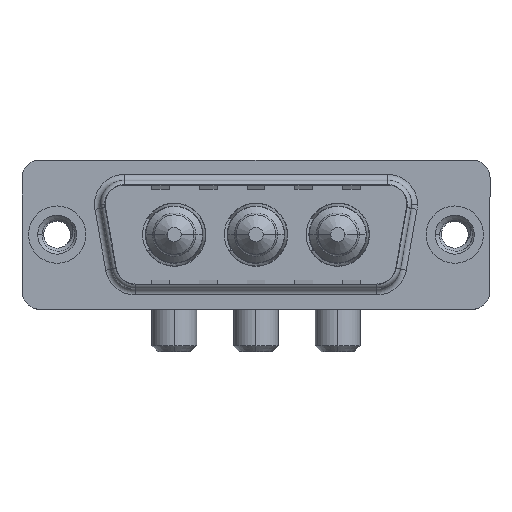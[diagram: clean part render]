
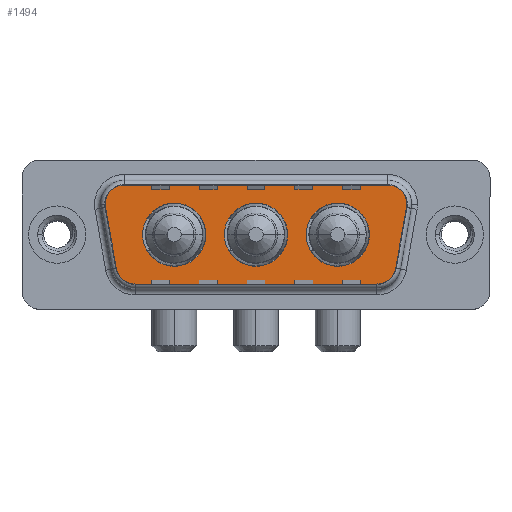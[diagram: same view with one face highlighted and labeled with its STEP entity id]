
A CAD part, top view. The second image highlights one B-rep face of the part: STEP entity #1494.
In plain terms, the highlighted planar face has unit normal (0, 0, 1).
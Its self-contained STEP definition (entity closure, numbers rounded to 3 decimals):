
#97 = ORIENTED_EDGE ( 'NONE', *, *, #5931, .T. ) ;
#112 = EDGE_LOOP ( 'NONE', ( #802, #237 ) ) ;
#126 = ORIENTED_EDGE ( 'NONE', *, *, #7953, .T. ) ;
#143 = CIRCLE ( 'NONE', #6179, 2.65 ) ;
#225 = FACE_BOUND ( 'NONE', #112, .T. ) ;
#237 = ORIENTED_EDGE ( 'NONE', *, *, #694, .F. ) ;
#276 = ORIENTED_EDGE ( 'NONE', *, *, #11775, .F. ) ;
#366 = EDGE_CURVE ( 'NONE', #3115, #2469, #8576, .T. ) ;
#438 = DIRECTION ( 'NONE',  ( 0., 0., 1. ) ) ;
#496 = CARTESIAN_POINT ( 'NONE',  ( 26.866, -2.9, 0. ) ) ;
#541 = CIRCLE ( 'NONE', #2817, 2. ) ;
#557 = DIRECTION ( 'NONE',  ( 1., 0., 0. ) ) ;
#694 = EDGE_CURVE ( 'NONE', #3726, #1870, #6298, .T. ) ;
#802 = ORIENTED_EDGE ( 'NONE', *, *, #11049, .F. ) ;
#808 = CARTESIAN_POINT ( 'NONE',  ( 23.5, 0., 0. ) ) ;
#925 = FACE_BOUND ( 'NONE', #8384, .T. ) ;
#1011 = CARTESIAN_POINT ( 'NONE',  ( 29.859, 2.553, 0. ) ) ;
#1080 = CIRCLE ( 'NONE', #6292, 2. ) ;
#1081 = CARTESIAN_POINT ( 'NONE',  ( 4.464, -3.247, 0. ) ) ;
#1180 = ORIENTED_EDGE ( 'NONE', *, *, #366, .T. ) ;
#1191 = CARTESIAN_POINT ( 'NONE',  ( 26.866, -2.9, 0. ) ) ;
#1372 = DIRECTION ( 'NONE',  ( 0., 0., 1. ) ) ;
#1472 = DIRECTION ( 'NONE',  ( 1., 0., 0. ) ) ;
#1494 = ADVANCED_FACE ( 'NONE', ( #10146, #925, #225, #2933 ), #9034, .T. ) ;
#1510 = ORIENTED_EDGE ( 'NONE', *, *, #2266, .T. ) ;
#1713 = AXIS2_PLACEMENT_3D ( 'NONE', #1191, #9162, #8184 ) ;
#1784 = AXIS2_PLACEMENT_3D ( 'NONE', #7742, #1927, #6703 ) ;
#1803 = AXIS2_PLACEMENT_3D ( 'NONE', #6799, #9805, #8179 ) ;
#1870 = VERTEX_POINT ( 'NONE', #9082 ) ;
#1927 = DIRECTION ( 'NONE',  ( 0., 0., 1. ) ) ;
#1985 = ORIENTED_EDGE ( 'NONE', *, *, #9459, .F. ) ;
#2036 = CARTESIAN_POINT ( 'NONE',  ( 27.889, 4.9, 0. ) ) ;
#2051 = VERTEX_POINT ( 'NONE', #4341 ) ;
#2266 = EDGE_CURVE ( 'NONE', #2051, #5206, #11802, .T. ) ;
#2469 = VERTEX_POINT ( 'NONE', #2036 ) ;
#2501 = DIRECTION ( 'NONE',  ( 0., 0., 1. ) ) ;
#2682 = DIRECTION ( 'NONE',  ( 0.174, -0.985, 0. ) ) ;
#2817 = AXIS2_PLACEMENT_3D ( 'NONE', #11311, #12238, #8225 ) ;
#2933 = FACE_OUTER_BOUND ( 'NONE', #5765, .T. ) ;
#2981 = CARTESIAN_POINT ( 'NONE',  ( 5.411, 4.9, 0. ) ) ;
#2986 = CARTESIAN_POINT ( 'NONE',  ( 5.411, 2.9, 0. ) ) ;
#3115 = VERTEX_POINT ( 'NONE', #12244 ) ;
#3294 = AXIS2_PLACEMENT_3D ( 'NONE', #808, #12917, #5832 ) ;
#3415 = VECTOR ( 'NONE', #2682, 1000. ) ;
#3726 = VERTEX_POINT ( 'NONE', #6502 ) ;
#4155 = DIRECTION ( 'NONE',  ( 0., 0., 1. ) ) ;
#4234 = EDGE_CURVE ( 'NONE', #7872, #2051, #11954, .T. ) ;
#4341 = CARTESIAN_POINT ( 'NONE',  ( 3.441, 2.553, 0. ) ) ;
#4369 = CARTESIAN_POINT ( 'NONE',  ( 20.85, 0., 0. ) ) ;
#4537 = DIRECTION ( 'NONE',  ( 1., 0., 0. ) ) ;
#4610 = ORIENTED_EDGE ( 'NONE', *, *, #10403, .T. ) ;
#4778 = VERTEX_POINT ( 'NONE', #6060 ) ;
#5125 = CIRCLE ( 'NONE', #6165, 2.65 ) ;
#5206 = VERTEX_POINT ( 'NONE', #1081 ) ;
#5215 = DIRECTION ( 'NONE',  ( -1., 0., 0. ) ) ;
#5291 = CARTESIAN_POINT ( 'NONE',  ( 27.889, 2.9, 0. ) ) ;
#5457 = EDGE_CURVE ( 'NONE', #4778, #12009, #1080, .T. ) ;
#5512 = CARTESIAN_POINT ( 'NONE',  ( 6.434, -4.9, 0. ) ) ;
#5677 = VECTOR ( 'NONE', #12750, 1000. ) ;
#5765 = EDGE_LOOP ( 'NONE', ( #12275, #97, #8215, #1180, #126, #8642, #1510, #4610, #12386 ) ) ;
#5774 = VECTOR ( 'NONE', #557, 1000. ) ;
#5832 = DIRECTION ( 'NONE',  ( 1., 0., 0. ) ) ;
#5931 = EDGE_CURVE ( 'NONE', #12009, #6503, #7456, .T. ) ;
#6060 = CARTESIAN_POINT ( 'NONE',  ( 26.866, -4.9, 0. ) ) ;
#6165 = AXIS2_PLACEMENT_3D ( 'NONE', #9311, #2501, #8082 ) ;
#6179 = AXIS2_PLACEMENT_3D ( 'NONE', #11361, #12417, #4537 ) ;
#6241 = DIRECTION ( 'NONE',  ( 1., 0., 0. ) ) ;
#6292 = AXIS2_PLACEMENT_3D ( 'NONE', #496, #11485, #12654 ) ;
#6298 = CIRCLE ( 'NONE', #6494, 2.65 ) ;
#6391 = CIRCLE ( 'NONE', #1784, 2. ) ;
#6456 = ORIENTED_EDGE ( 'NONE', *, *, #12552, .F. ) ;
#6476 = CARTESIAN_POINT ( 'NONE',  ( 29.859, 2.553, 0. ) ) ;
#6494 = AXIS2_PLACEMENT_3D ( 'NONE', #9323, #438, #1472 ) ;
#6502 = CARTESIAN_POINT ( 'NONE',  ( 7.15, 0., 0. ) ) ;
#6503 = VERTEX_POINT ( 'NONE', #1011 ) ;
#6703 = DIRECTION ( 'NONE',  ( -1., 0., 0. ) ) ;
#6799 = CARTESIAN_POINT ( 'NONE',  ( 23.5, 0., 0. ) ) ;
#6870 = EDGE_LOOP ( 'NONE', ( #1985, #7999 ) ) ;
#7189 = VERTEX_POINT ( 'NONE', #8636 ) ;
#7347 = LINE ( 'NONE', #5512, #5774 ) ;
#7456 = LINE ( 'NONE', #6476, #5677 ) ;
#7674 = CIRCLE ( 'NONE', #3294, 2.65 ) ;
#7742 = CARTESIAN_POINT ( 'NONE',  ( 27.889, 2.9, 0. ) ) ;
#7860 = VERTEX_POINT ( 'NONE', #11845 ) ;
#7872 = VERTEX_POINT ( 'NONE', #2981 ) ;
#7953 = EDGE_CURVE ( 'NONE', #2469, #7872, #11120, .T. ) ;
#7999 = ORIENTED_EDGE ( 'NONE', *, *, #8372, .F. ) ;
#8019 = VERTEX_POINT ( 'NONE', #4369 ) ;
#8031 = DIRECTION ( 'NONE',  ( 1., 0., 0. ) ) ;
#8082 = DIRECTION ( 'NONE',  ( 1., 0., 0. ) ) ;
#8141 = CARTESIAN_POINT ( 'NONE',  ( 16.65, 0., 0. ) ) ;
#8162 = CARTESIAN_POINT ( 'NONE',  ( 5.411, 4.9, 0. ) ) ;
#8179 = DIRECTION ( 'NONE',  ( 1., 0., 0. ) ) ;
#8184 = DIRECTION ( 'NONE',  ( 1., 0., 0. ) ) ;
#8215 = ORIENTED_EDGE ( 'NONE', *, *, #10777, .T. ) ;
#8225 = DIRECTION ( 'NONE',  ( -1., 0., 0. ) ) ;
#8372 = EDGE_CURVE ( 'NONE', #7189, #7860, #5125, .T. ) ;
#8384 = EDGE_LOOP ( 'NONE', ( #276, #6456 ) ) ;
#8438 = VERTEX_POINT ( 'NONE', #12344 ) ;
#8576 = CIRCLE ( 'NONE', #10492, 2. ) ;
#8598 = CARTESIAN_POINT ( 'NONE',  ( 28.836, -3.247, 0. ) ) ;
#8636 = CARTESIAN_POINT ( 'NONE',  ( 14., 0., 0. ) ) ;
#8642 = ORIENTED_EDGE ( 'NONE', *, *, #4234, .T. ) ;
#8954 = DIRECTION ( 'NONE',  ( 0., 0., 1. ) ) ;
#8979 = CARTESIAN_POINT ( 'NONE',  ( 26.15, 0., 0. ) ) ;
#9034 = PLANE ( 'NONE',  #1713 ) ;
#9082 = CARTESIAN_POINT ( 'NONE',  ( 12.45, 0., 0. ) ) ;
#9158 = DIRECTION ( 'NONE',  ( -1., 0., 0. ) ) ;
#9162 = DIRECTION ( 'NONE',  ( 0., 0., 1. ) ) ;
#9311 = CARTESIAN_POINT ( 'NONE',  ( 16.65, 0., 0. ) ) ;
#9323 = CARTESIAN_POINT ( 'NONE',  ( 9.8, 0., 0. ) ) ;
#9459 = EDGE_CURVE ( 'NONE', #7860, #7189, #10167, .T. ) ;
#9499 = VECTOR ( 'NONE', #5215, 1000. ) ;
#9638 = AXIS2_PLACEMENT_3D ( 'NONE', #2986, #8954, #8031 ) ;
#9681 = EDGE_CURVE ( 'NONE', #8438, #4778, #7347, .T. ) ;
#9805 = DIRECTION ( 'NONE',  ( 0., 0., 1. ) ) ;
#10146 = FACE_BOUND ( 'NONE', #6870, .T. ) ;
#10167 = CIRCLE ( 'NONE', #11215, 2.65 ) ;
#10403 = EDGE_CURVE ( 'NONE', #5206, #8438, #541, .T. ) ;
#10492 = AXIS2_PLACEMENT_3D ( 'NONE', #5291, #1372, #9158 ) ;
#10777 = EDGE_CURVE ( 'NONE', #6503, #3115, #6391, .T. ) ;
#11049 = EDGE_CURVE ( 'NONE', #1870, #3726, #143, .T. ) ;
#11120 = LINE ( 'NONE', #8162, #9499 ) ;
#11215 = AXIS2_PLACEMENT_3D ( 'NONE', #8141, #4155, #6241 ) ;
#11311 = CARTESIAN_POINT ( 'NONE',  ( 6.434, -2.9, 0. ) ) ;
#11361 = CARTESIAN_POINT ( 'NONE',  ( 9.8, 0., 0. ) ) ;
#11404 = VERTEX_POINT ( 'NONE', #8979 ) ;
#11485 = DIRECTION ( 'NONE',  ( 0., 0., 1. ) ) ;
#11775 = EDGE_CURVE ( 'NONE', #11404, #8019, #12488, .T. ) ;
#11802 = LINE ( 'NONE', #12531, #3415 ) ;
#11845 = CARTESIAN_POINT ( 'NONE',  ( 19.3, 0., 0. ) ) ;
#11954 = CIRCLE ( 'NONE', #9638, 2. ) ;
#12009 = VERTEX_POINT ( 'NONE', #8598 ) ;
#12238 = DIRECTION ( 'NONE',  ( 0., 0., 1. ) ) ;
#12244 = CARTESIAN_POINT ( 'NONE',  ( 29.889, 2.9, 0. ) ) ;
#12275 = ORIENTED_EDGE ( 'NONE', *, *, #5457, .T. ) ;
#12344 = CARTESIAN_POINT ( 'NONE',  ( 6.434, -4.9, 0. ) ) ;
#12386 = ORIENTED_EDGE ( 'NONE', *, *, #9681, .T. ) ;
#12417 = DIRECTION ( 'NONE',  ( 0., 0., 1. ) ) ;
#12488 = CIRCLE ( 'NONE', #1803, 2.65 ) ;
#12531 = CARTESIAN_POINT ( 'NONE',  ( 3.441, 2.553, 0. ) ) ;
#12552 = EDGE_CURVE ( 'NONE', #8019, #11404, #7674, .T. ) ;
#12654 = DIRECTION ( 'NONE',  ( 1., 0., 0. ) ) ;
#12750 = DIRECTION ( 'NONE',  ( 0.174, 0.985, 0. ) ) ;
#12917 = DIRECTION ( 'NONE',  ( 0., 0., 1. ) ) ;
